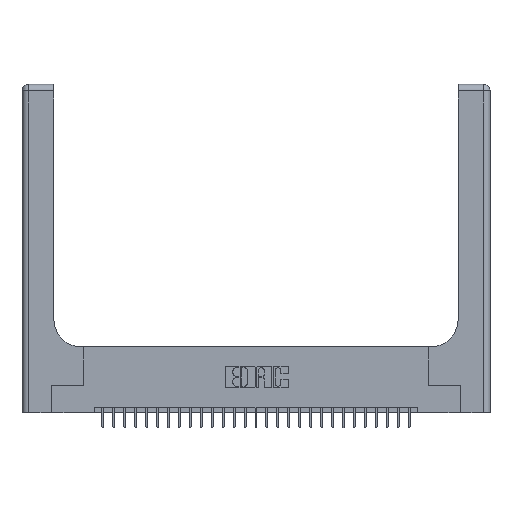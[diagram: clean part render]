
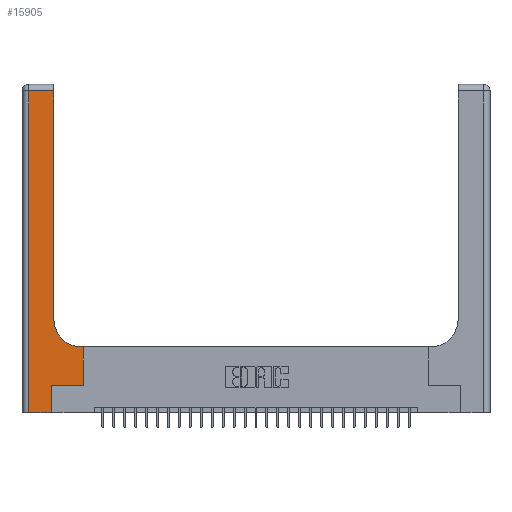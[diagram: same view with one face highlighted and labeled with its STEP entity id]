
A CAD part, top view. The second image highlights one B-rep face of the part: STEP entity #15905.
In plain terms, the highlighted planar face has unit normal (0, 0, 1).
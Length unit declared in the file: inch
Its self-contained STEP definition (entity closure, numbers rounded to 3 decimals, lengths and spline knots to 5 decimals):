
#116 = DIRECTION ( 'NONE',  ( 0., 1., 0. ) ) ;
#266 = ORIENTED_EDGE ( 'NONE', *, *, #6933, .T. ) ;
#281 = LINE ( 'NONE', #16416, #12587 ) ;
#407 = CARTESIAN_POINT ( 'NONE',  ( 0.2915, 3., 0.37 ) ) ;
#486 = EDGE_CURVE ( 'NONE', #17117, #18870, #20638, .T. ) ;
#870 = DIRECTION ( 'NONE',  ( 1., 0., 0. ) ) ;
#2050 = ORIENTED_EDGE ( 'NONE', *, *, #15457, .T. ) ;
#2063 = CARTESIAN_POINT ( 'NONE',  ( 0.5585, 0.6, 0.37 ) ) ;
#2703 = DIRECTION ( 'NONE',  ( 1., 0., 0. ) ) ;
#2923 = ORIENTED_EDGE ( 'NONE', *, *, #23212, .T. ) ;
#2978 = DIRECTION ( 'NONE',  ( 0., 1., 0. ) ) ;
#3234 = LINE ( 'NONE', #23766, #10069 ) ;
#3429 = DIRECTION ( 'NONE',  ( 0., 0., -1. ) ) ;
#3540 = DIRECTION ( 'NONE',  ( 0., -1., 0. ) ) ;
#3559 = DIRECTION ( 'NONE',  ( 0., 0., -1. ) ) ;
#3603 = VECTOR ( 'NONE', #23218, 39.37008 ) ;
#4632 = EDGE_CURVE ( 'NONE', #14005, #17117, #19311, .T. ) ;
#4769 = CARTESIAN_POINT ( 'NONE',  ( 0.06, 0., 0.37 ) ) ;
#4785 = CARTESIAN_POINT ( 'NONE',  ( 0.2915, 0.6, 0.37 ) ) ;
#5936 = EDGE_CURVE ( 'NONE', #29227, #14005, #9294, .T. ) ;
#6100 = EDGE_CURVE ( 'NONE', #27981, #19040, #22620, .T. ) ;
#6295 = AXIS2_PLACEMENT_3D ( 'NONE', #12452, #3559, #870 ) ;
#6933 = EDGE_CURVE ( 'NONE', #16790, #22389, #11317, .T. ) ;
#6954 = CARTESIAN_POINT ( 'NONE',  ( 0.269, 0.25, 0.37 ) ) ;
#7507 = ORIENTED_EDGE ( 'NONE', *, *, #6100, .T. ) ;
#7628 = CARTESIAN_POINT ( 'NONE',  ( 0.2915, 2.94, 0.37 ) ) ;
#7922 = CARTESIAN_POINT ( 'NONE',  ( 0.269, 0., 0.37 ) ) ;
#8033 = AXIS2_PLACEMENT_3D ( 'NONE', #17004, #3429, #12314 ) ;
#9294 = LINE ( 'NONE', #4785, #3603 ) ;
#10042 = PLANE ( 'NONE',  #8033 ) ;
#10044 = LINE ( 'NONE', #12624, #24852 ) ;
#10069 = VECTOR ( 'NONE', #3540, 39.37008 ) ;
#10084 = ORIENTED_EDGE ( 'NONE', *, *, #486, .T. ) ;
#10193 = FACE_OUTER_BOUND ( 'NONE', #14786, .T. ) ;
#10579 = CARTESIAN_POINT ( 'NONE',  ( 0.5585, 0.25, 0.37 ) ) ;
#11317 = LINE ( 'NONE', #23256, #26886 ) ;
#12314 = DIRECTION ( 'NONE',  ( -1., 0., 0. ) ) ;
#12452 = CARTESIAN_POINT ( 'NONE',  ( 0.5415, 0.85, 0.37 ) ) ;
#12499 = DIRECTION ( 'NONE',  ( -1., 0., 0. ) ) ;
#12587 = VECTOR ( 'NONE', #20514, 39.37008 ) ;
#12624 = CARTESIAN_POINT ( 'NONE',  ( 0.5585, 0.25, 0.37 ) ) ;
#13425 = CARTESIAN_POINT ( 'NONE',  ( 0.5415, 0.6, 0.37 ) ) ;
#14005 = VERTEX_POINT ( 'NONE', #13425 ) ;
#14710 = VECTOR ( 'NONE', #15963, 39.37008 ) ;
#14786 = EDGE_LOOP ( 'NONE', ( #10084, #2050, #16472, #7507, #2923, #266, #27066, #20213, #15921 ) ) ;
#15457 = EDGE_CURVE ( 'NONE', #18870, #16079, #24140, .T. ) ;
#15905 = ADVANCED_FACE ( 'NONE', ( #10193 ), #10042, .F. ) ;
#15921 = ORIENTED_EDGE ( 'NONE', *, *, #4632, .T. ) ;
#15963 = DIRECTION ( 'NONE',  ( 1., 0., 0. ) ) ;
#16079 = VERTEX_POINT ( 'NONE', #29363 ) ;
#16416 = CARTESIAN_POINT ( 'NONE',  ( 0.269, 0., 0.37 ) ) ;
#16472 = ORIENTED_EDGE ( 'NONE', *, *, #20747, .T. ) ;
#16790 = VERTEX_POINT ( 'NONE', #6954 ) ;
#17004 = CARTESIAN_POINT ( 'NONE',  ( 0., 3., 0.37 ) ) ;
#17117 = VERTEX_POINT ( 'NONE', #25192 ) ;
#18068 = CARTESIAN_POINT ( 'NONE',  ( 0., 0., 0.37 ) ) ;
#18870 = VERTEX_POINT ( 'NONE', #7628 ) ;
#19040 = VERTEX_POINT ( 'NONE', #7922 ) ;
#19311 = CIRCLE ( 'NONE', #6295, 0.25 ) ;
#19462 = CARTESIAN_POINT ( 'NONE',  ( 0., 2.94, 0.37 ) ) ;
#20213 = ORIENTED_EDGE ( 'NONE', *, *, #5936, .T. ) ;
#20514 = DIRECTION ( 'NONE',  ( 0., 1., 0. ) ) ;
#20638 = LINE ( 'NONE', #407, #26376 ) ;
#20747 = EDGE_CURVE ( 'NONE', #16079, #27981, #3234, .T. ) ;
#22389 = VERTEX_POINT ( 'NONE', #10579 ) ;
#22620 = LINE ( 'NONE', #18068, #14710 ) ;
#23212 = EDGE_CURVE ( 'NONE', #19040, #16790, #281, .T. ) ;
#23218 = DIRECTION ( 'NONE',  ( -1., 0., 0. ) ) ;
#23256 = CARTESIAN_POINT ( 'NONE',  ( 0.269, 0.25, 0.37 ) ) ;
#23766 = CARTESIAN_POINT ( 'NONE',  ( 0.06, 3., 0.37 ) ) ;
#24140 = LINE ( 'NONE', #19462, #26338 ) ;
#24668 = EDGE_CURVE ( 'NONE', #22389, #29227, #10044, .T. ) ;
#24852 = VECTOR ( 'NONE', #2978, 39.37008 ) ;
#25192 = CARTESIAN_POINT ( 'NONE',  ( 0.2915, 0.85, 0.37 ) ) ;
#26338 = VECTOR ( 'NONE', #12499, 39.37008 ) ;
#26376 = VECTOR ( 'NONE', #116, 39.37008 ) ;
#26886 = VECTOR ( 'NONE', #2703, 39.37008 ) ;
#27066 = ORIENTED_EDGE ( 'NONE', *, *, #24668, .T. ) ;
#27981 = VERTEX_POINT ( 'NONE', #4769 ) ;
#29227 = VERTEX_POINT ( 'NONE', #2063 ) ;
#29363 = CARTESIAN_POINT ( 'NONE',  ( 0.06, 2.94, 0.37 ) ) ;
